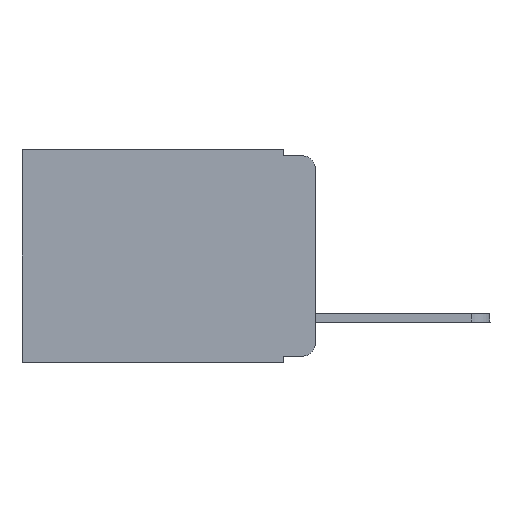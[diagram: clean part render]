
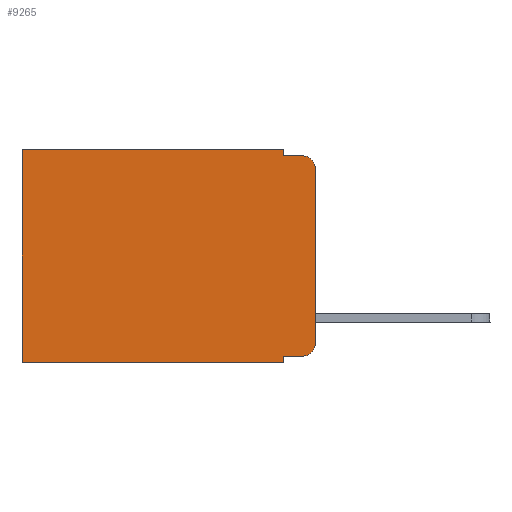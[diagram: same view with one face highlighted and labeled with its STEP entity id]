
A CAD part, left-side view. The second image highlights one B-rep face of the part: STEP entity #9265.
In plain terms, the highlighted planar face has unit normal (-1, 0, 0).
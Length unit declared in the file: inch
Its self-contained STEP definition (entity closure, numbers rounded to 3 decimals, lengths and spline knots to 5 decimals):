
#134 = DIRECTION ( 'NONE',  ( -1., 0., 0. ) ) ;
#287 = ORIENTED_EDGE ( 'NONE', *, *, #404, .F. ) ;
#404 = EDGE_CURVE ( 'NONE', #14623, #6995, #4163, .T. ) ;
#533 = CARTESIAN_POINT ( 'NONE',  ( 0.298, 0.051, 0. ) ) ;
#592 = DIRECTION ( 'NONE',  ( 0., 0., -1. ) ) ;
#683 = DIRECTION ( 'NONE',  ( 0., 0., -1. ) ) ;
#764 = VECTOR ( 'NONE', #11602, 39.37008 ) ;
#1017 = VERTEX_POINT ( 'NONE', #4420 ) ;
#1400 = CIRCLE ( 'NONE', #5925, 0.02 ) ;
#1635 = CARTESIAN_POINT ( 'NONE',  ( 0.298, 0., 0. ) ) ;
#1953 = DIRECTION ( 'NONE',  ( -1., 0., 0. ) ) ;
#2164 = CARTESIAN_POINT ( 'NONE',  ( 0.298, 0.473, -0.343 ) ) ;
#2228 = CARTESIAN_POINT ( 'NONE',  ( 0.298, 0.051, -0.333 ) ) ;
#2500 = AXIS2_PLACEMENT_3D ( 'NONE', #7595, #1953, #10099 ) ;
#2791 = CARTESIAN_POINT ( 'NONE',  ( 0.298, 0.051, -0.01 ) ) ;
#3557 = ORIENTED_EDGE ( 'NONE', *, *, #8326, .T. ) ;
#3722 = EDGE_CURVE ( 'NONE', #14047, #11545, #10800, .T. ) ;
#4013 = VECTOR ( 'NONE', #7645, 39.37008 ) ;
#4125 = CARTESIAN_POINT ( 'NONE',  ( 0.298, 0., 0. ) ) ;
#4163 = LINE ( 'NONE', #12649, #13647 ) ;
#4203 = ORIENTED_EDGE ( 'NONE', *, *, #12387, .F. ) ;
#4420 = CARTESIAN_POINT ( 'NONE',  ( 0.298, 0., -0.313 ) ) ;
#4640 = VECTOR ( 'NONE', #683, 39.37008 ) ;
#4641 = CARTESIAN_POINT ( 'NONE',  ( 0.298, 0.02, -0.03 ) ) ;
#4749 = AXIS2_PLACEMENT_3D ( 'NONE', #5164, #6086, #7272 ) ;
#4764 = CARTESIAN_POINT ( 'NONE',  ( 0.298, 0.02, -0.333 ) ) ;
#5009 = VERTEX_POINT ( 'NONE', #14029 ) ;
#5164 = CARTESIAN_POINT ( 'NONE',  ( 0.298, 0., 0. ) ) ;
#5638 = ORIENTED_EDGE ( 'NONE', *, *, #13486, .F. ) ;
#5925 = AXIS2_PLACEMENT_3D ( 'NONE', #4641, #134, #10619 ) ;
#6086 = DIRECTION ( 'NONE',  ( 1., 0., 0. ) ) ;
#6200 = EDGE_CURVE ( 'NONE', #14047, #14421, #13676, .T. ) ;
#6210 = CARTESIAN_POINT ( 'NONE',  ( 0.298, 0.051, 0. ) ) ;
#6461 = VECTOR ( 'NONE', #7193, 39.37008 ) ;
#6579 = CARTESIAN_POINT ( 'NONE',  ( 0.298, 0.051, 0. ) ) ;
#6670 = ORIENTED_EDGE ( 'NONE', *, *, #14754, .F. ) ;
#6890 = VECTOR ( 'NONE', #592, 39.37008 ) ;
#6995 = VERTEX_POINT ( 'NONE', #10525 ) ;
#7193 = DIRECTION ( 'NONE',  ( 0., 0., -1. ) ) ;
#7272 = DIRECTION ( 'NONE',  ( 0., 0., -1. ) ) ;
#7595 = CARTESIAN_POINT ( 'NONE',  ( 0.298, 0.02, -0.313 ) ) ;
#7645 = DIRECTION ( 'NONE',  ( 0., 0., -1. ) ) ;
#7804 = VERTEX_POINT ( 'NONE', #11986 ) ;
#7874 = FACE_OUTER_BOUND ( 'NONE', #10179, .T. ) ;
#8291 = LINE ( 'NONE', #14130, #6461 ) ;
#8326 = EDGE_CURVE ( 'NONE', #7804, #9481, #8291, .T. ) ;
#8555 = EDGE_CURVE ( 'NONE', #12184, #7804, #14503, .T. ) ;
#8631 = PLANE ( 'NONE',  #4749 ) ;
#9198 = DIRECTION ( 'NONE',  ( 0., -1., 0. ) ) ;
#9265 = ADVANCED_FACE ( 'NONE', ( #7874 ), #8631, .F. ) ;
#9481 = VERTEX_POINT ( 'NONE', #2164 ) ;
#10006 = ORIENTED_EDGE ( 'NONE', *, *, #3722, .T. ) ;
#10072 = EDGE_CURVE ( 'NONE', #11545, #1017, #10761, .T. ) ;
#10099 = DIRECTION ( 'NONE',  ( 0., 0., -1. ) ) ;
#10179 = EDGE_LOOP ( 'NONE', ( #6670, #10583, #287, #4203, #13385, #3557, #5638, #10961, #10006, #13473 ) ) ;
#10525 = CARTESIAN_POINT ( 'NONE',  ( 0.298, 0.02, -0.01 ) ) ;
#10583 = ORIENTED_EDGE ( 'NONE', *, *, #12646, .T. ) ;
#10619 = DIRECTION ( 'NONE',  ( 0., 0., -1. ) ) ;
#10761 = CIRCLE ( 'NONE', #2500, 0.02 ) ;
#10800 = LINE ( 'NONE', #2228, #764 ) ;
#10939 = DIRECTION ( 'NONE',  ( 0., 1., 0. ) ) ;
#10961 = ORIENTED_EDGE ( 'NONE', *, *, #6200, .F. ) ;
#11019 = CARTESIAN_POINT ( 'NONE',  ( 0.298, 0., -0.343 ) ) ;
#11020 = LINE ( 'NONE', #11019, #12115 ) ;
#11414 = CARTESIAN_POINT ( 'NONE',  ( 0.298, 0.051, -0.343 ) ) ;
#11545 = VERTEX_POINT ( 'NONE', #4764 ) ;
#11602 = DIRECTION ( 'NONE',  ( 0., -1., 0. ) ) ;
#11986 = CARTESIAN_POINT ( 'NONE',  ( 0.298, 0.473, 0. ) ) ;
#12115 = VECTOR ( 'NONE', #13167, 39.37008 ) ;
#12184 = VERTEX_POINT ( 'NONE', #6210 ) ;
#12387 = EDGE_CURVE ( 'NONE', #12184, #14623, #13990, .T. ) ;
#12646 = EDGE_CURVE ( 'NONE', #5009, #6995, #1400, .T. ) ;
#12649 = CARTESIAN_POINT ( 'NONE',  ( 0.298, 0.051, -0.01 ) ) ;
#13167 = DIRECTION ( 'NONE',  ( 0., 1., 0. ) ) ;
#13200 = CARTESIAN_POINT ( 'NONE',  ( 0.298, 0.051, -0.333 ) ) ;
#13385 = ORIENTED_EDGE ( 'NONE', *, *, #8555, .T. ) ;
#13473 = ORIENTED_EDGE ( 'NONE', *, *, #10072, .T. ) ;
#13486 = EDGE_CURVE ( 'NONE', #14421, #9481, #11020, .T. ) ;
#13647 = VECTOR ( 'NONE', #9198, 39.37008 ) ;
#13676 = LINE ( 'NONE', #6579, #4013 ) ;
#13937 = LINE ( 'NONE', #4125, #4640 ) ;
#13990 = LINE ( 'NONE', #533, #6890 ) ;
#14029 = CARTESIAN_POINT ( 'NONE',  ( 0.298, 0., -0.03 ) ) ;
#14047 = VERTEX_POINT ( 'NONE', #13200 ) ;
#14130 = CARTESIAN_POINT ( 'NONE',  ( 0.298, 0.473, 0. ) ) ;
#14421 = VERTEX_POINT ( 'NONE', #11414 ) ;
#14503 = LINE ( 'NONE', #1635, #14690 ) ;
#14623 = VERTEX_POINT ( 'NONE', #2791 ) ;
#14690 = VECTOR ( 'NONE', #10939, 39.37008 ) ;
#14754 = EDGE_CURVE ( 'NONE', #5009, #1017, #13937, .T. ) ;
